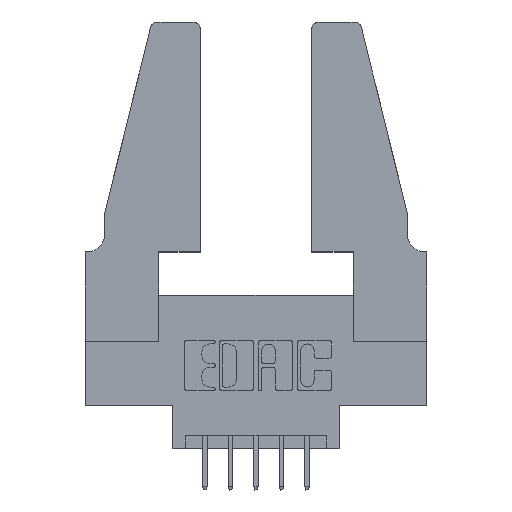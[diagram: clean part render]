
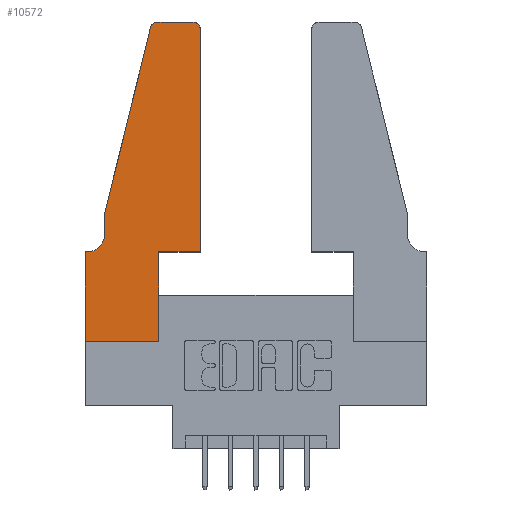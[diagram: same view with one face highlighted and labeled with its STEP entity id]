
A CAD part, top view. The second image highlights one B-rep face of the part: STEP entity #10572.
In plain terms, the highlighted planar face has unit normal (0, 0, 1).
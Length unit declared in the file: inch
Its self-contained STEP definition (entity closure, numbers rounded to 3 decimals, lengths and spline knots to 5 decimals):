
#73 = VERTEX_POINT ( 'NONE', #8285 ) ;
#169 = CARTESIAN_POINT ( 'NONE',  ( 0., 0.35, 0.37 ) ) ;
#203 = CIRCLE ( 'NONE', #1934, 0.03 ) ;
#278 = ORIENTED_EDGE ( 'NONE', *, *, #7301, .T. ) ;
#411 = FACE_OUTER_BOUND ( 'NONE', #6222, .T. ) ;
#427 = CARTESIAN_POINT ( 'NONE',  ( 0.0755, 0.35, 0.37 ) ) ;
#482 = CARTESIAN_POINT ( 'NONE',  ( 0.4505, 0.35, 0.37 ) ) ;
#742 = CARTESIAN_POINT ( 'NONE',  ( 0.0755, 0.42, 0.37 ) ) ;
#890 = CIRCLE ( 'NONE', #6960, 0.03 ) ;
#1268 = VERTEX_POINT ( 'NONE', #10892 ) ;
#1448 = DIRECTION ( 'NONE',  ( 0., 1., 0. ) ) ;
#1490 = VERTEX_POINT ( 'NONE', #4712 ) ;
#1499 = VERTEX_POINT ( 'NONE', #5498 ) ;
#1512 = ORIENTED_EDGE ( 'NONE', *, *, #10780, .T. ) ;
#1547 = LINE ( 'NONE', #10992, #6434 ) ;
#1734 = VECTOR ( 'NONE', #3119, 39.37008 ) ;
#1788 = LINE ( 'NONE', #10891, #6541 ) ;
#1810 = VERTEX_POINT ( 'NONE', #10895 ) ;
#1868 = LINE ( 'NONE', #3410, #7305 ) ;
#1934 = AXIS2_PLACEMENT_3D ( 'NONE', #9405, #10449, #6842 ) ;
#2189 = ORIENTED_EDGE ( 'NONE', *, *, #10944, .T. ) ;
#2361 = ORIENTED_EDGE ( 'NONE', *, *, #2569, .T. ) ;
#2391 = PLANE ( 'NONE',  #11191 ) ;
#2393 = CARTESIAN_POINT ( 'NONE',  ( 0., 0., 0.37 ) ) ;
#2542 = EDGE_CURVE ( 'NONE', #5766, #7526, #5526, .T. ) ;
#2569 = EDGE_CURVE ( 'NONE', #1490, #1268, #10994, .T. ) ;
#2606 = ORIENTED_EDGE ( 'NONE', *, *, #5325, .T. ) ;
#2713 = LINE ( 'NONE', #427, #7614 ) ;
#3119 = DIRECTION ( 'NONE',  ( 1., 0., 0. ) ) ;
#3132 = ORIENTED_EDGE ( 'NONE', *, *, #2542, .T. ) ;
#3373 = DIRECTION ( 'NONE',  ( 0., 0., 1. ) ) ;
#3410 = CARTESIAN_POINT ( 'NONE',  ( 0.0755, 0.5, 0.37 ) ) ;
#3468 = EDGE_CURVE ( 'NONE', #4893, #73, #1547, .T. ) ;
#3547 = VERTEX_POINT ( 'NONE', #6977 ) ;
#3631 = EDGE_CURVE ( 'NONE', #1810, #6019, #890, .T. ) ;
#3650 = DIRECTION ( 'NONE',  ( 0., 0., 1. ) ) ;
#3746 = AXIS2_PLACEMENT_3D ( 'NONE', #6338, #10789, #4663 ) ;
#3852 = VERTEX_POINT ( 'NONE', #7428 ) ;
#4039 = VECTOR ( 'NONE', #9199, 39.37008 ) ;
#4307 = EDGE_CURVE ( 'NONE', #73, #3852, #203, .T. ) ;
#4663 = DIRECTION ( 'NONE',  ( -1., 0., 0. ) ) ;
#4669 = CARTESIAN_POINT ( 'NONE',  ( 0.2605, 1.25, 0.37 ) ) ;
#4712 = CARTESIAN_POINT ( 'NONE',  ( 0.2865, 0., 0.37 ) ) ;
#4893 = VERTEX_POINT ( 'NONE', #6886 ) ;
#5325 = EDGE_CURVE ( 'NONE', #7526, #1490, #1788, .T. ) ;
#5498 = CARTESIAN_POINT ( 'NONE',  ( 0.0755, 0.5, 0.37 ) ) ;
#5526 = LINE ( 'NONE', #2393, #6066 ) ;
#5766 = VERTEX_POINT ( 'NONE', #169 ) ;
#5909 = ORIENTED_EDGE ( 'NONE', *, *, #4307, .T. ) ;
#5940 = EDGE_CURVE ( 'NONE', #3547, #5766, #2713, .T. ) ;
#6019 = VERTEX_POINT ( 'NONE', #11001 ) ;
#6066 = VECTOR ( 'NONE', #8486, 39.37008 ) ;
#6222 = EDGE_LOOP ( 'NONE', ( #8292, #8868, #8617, #278, #1512, #10025, #3132, #2606, #2361, #2189, #10112, #5909 ) ) ;
#6338 = CARTESIAN_POINT ( 'NONE',  ( 0.0055, 0.42, 0.37 ) ) ;
#6419 = DIRECTION ( 'NONE',  ( -1., 0., 0. ) ) ;
#6434 = VECTOR ( 'NONE', #1448, 39.37008 ) ;
#6444 = CARTESIAN_POINT ( 'NONE',  ( 0.0755, 0.5, 0.37 ) ) ;
#6500 = CIRCLE ( 'NONE', #3746, 0.07 ) ;
#6521 = DIRECTION ( 'NONE',  ( -1., 0., 0. ) ) ;
#6541 = VECTOR ( 'NONE', #9226, 39.37008 ) ;
#6842 = DIRECTION ( 'NONE',  ( 1., 0., 0. ) ) ;
#6886 = CARTESIAN_POINT ( 'NONE',  ( 0.4505, 0.35, 0.37 ) ) ;
#6960 = AXIS2_PLACEMENT_3D ( 'NONE', #10694, #3650, #9653 ) ;
#6977 = CARTESIAN_POINT ( 'NONE',  ( 0.0055, 0.35, 0.37 ) ) ;
#7050 = LINE ( 'NONE', #6444, #7184 ) ;
#7184 = VECTOR ( 'NONE', #10216, 39.37008 ) ;
#7301 = EDGE_CURVE ( 'NONE', #1499, #9133, #1868, .T. ) ;
#7305 = VECTOR ( 'NONE', #9486, 39.37008 ) ;
#7428 = CARTESIAN_POINT ( 'NONE',  ( 0.4205, 1.25, 0.37 ) ) ;
#7526 = VERTEX_POINT ( 'NONE', #9797 ) ;
#7614 = VECTOR ( 'NONE', #6521, 39.37008 ) ;
#7667 = EDGE_CURVE ( 'NONE', #6019, #1499, #7050, .T. ) ;
#8285 = CARTESIAN_POINT ( 'NONE',  ( 0.4505, 1.22, 0.37 ) ) ;
#8292 = ORIENTED_EDGE ( 'NONE', *, *, #8844, .T. ) ;
#8486 = DIRECTION ( 'NONE',  ( 0., -1., 0. ) ) ;
#8617 = ORIENTED_EDGE ( 'NONE', *, *, #7667, .T. ) ;
#8640 = DIRECTION ( 'NONE',  ( 1., 0., 0. ) ) ;
#8810 = LINE ( 'NONE', #482, #1734 ) ;
#8844 = EDGE_CURVE ( 'NONE', #3852, #1810, #8872, .T. ) ;
#8865 = CARTESIAN_POINT ( 'NONE',  ( 0.2865, 0.35, 0.37 ) ) ;
#8868 = ORIENTED_EDGE ( 'NONE', *, *, #3631, .T. ) ;
#8872 = LINE ( 'NONE', #4669, #10933 ) ;
#9133 = VERTEX_POINT ( 'NONE', #742 ) ;
#9199 = DIRECTION ( 'NONE',  ( 0., 1., 0. ) ) ;
#9226 = DIRECTION ( 'NONE',  ( 1., 0., 0. ) ) ;
#9405 = CARTESIAN_POINT ( 'NONE',  ( 0.4205, 1.22, 0.37 ) ) ;
#9417 = CARTESIAN_POINT ( 'NONE',  ( 0., 0.35, 0.37 ) ) ;
#9486 = DIRECTION ( 'NONE',  ( 0., -1., 0. ) ) ;
#9653 = DIRECTION ( 'NONE',  ( 1., 0., 0. ) ) ;
#9797 = CARTESIAN_POINT ( 'NONE',  ( 0., 0., 0.37 ) ) ;
#10025 = ORIENTED_EDGE ( 'NONE', *, *, #5940, .T. ) ;
#10112 = ORIENTED_EDGE ( 'NONE', *, *, #3468, .T. ) ;
#10216 = DIRECTION ( 'NONE',  ( -0.239, -0.971, 0. ) ) ;
#10449 = DIRECTION ( 'NONE',  ( 0., 0., 1. ) ) ;
#10572 = ADVANCED_FACE ( 'NONE', ( #411 ), #2391, .T. ) ;
#10694 = CARTESIAN_POINT ( 'NONE',  ( 0.284, 1.22, 0.37 ) ) ;
#10780 = EDGE_CURVE ( 'NONE', #9133, #3547, #6500, .T. ) ;
#10789 = DIRECTION ( 'NONE',  ( 0., 0., -1. ) ) ;
#10891 = CARTESIAN_POINT ( 'NONE',  ( 0., 0., 0.37 ) ) ;
#10892 = CARTESIAN_POINT ( 'NONE',  ( 0.2865, 0.35, 0.37 ) ) ;
#10895 = CARTESIAN_POINT ( 'NONE',  ( 0.284, 1.25, 0.37 ) ) ;
#10933 = VECTOR ( 'NONE', #6419, 39.37008 ) ;
#10944 = EDGE_CURVE ( 'NONE', #1268, #4893, #8810, .T. ) ;
#10992 = CARTESIAN_POINT ( 'NONE',  ( 0.4505, 0.35, 0.37 ) ) ;
#10994 = LINE ( 'NONE', #8865, #4039 ) ;
#11001 = CARTESIAN_POINT ( 'NONE',  ( 0.25487, 1.22718, 0.37 ) ) ;
#11191 = AXIS2_PLACEMENT_3D ( 'NONE', #9417, #3373, #8640 ) ;
